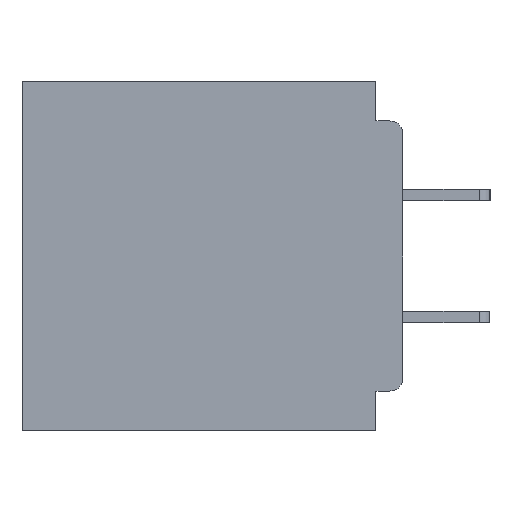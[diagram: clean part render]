
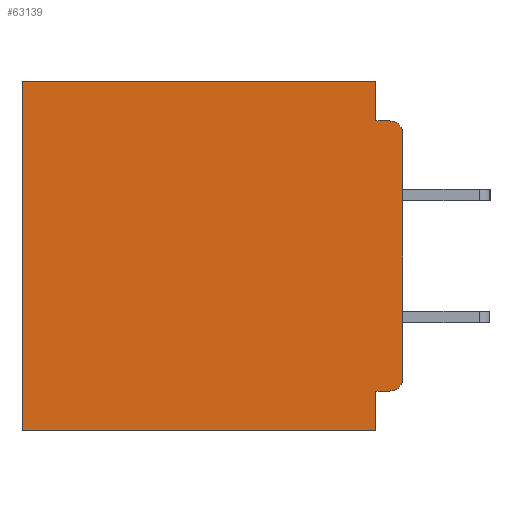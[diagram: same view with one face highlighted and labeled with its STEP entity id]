
A CAD part, left-side view. The second image highlights one B-rep face of the part: STEP entity #63139.
In plain terms, the highlighted planar face has unit normal (-1, 0, 0).
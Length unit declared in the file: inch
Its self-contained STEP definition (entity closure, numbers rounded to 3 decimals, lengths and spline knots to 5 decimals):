
#1406 = ORIENTED_EDGE ( 'NONE', *, *, #25688, .F. ) ;
#1884 = VERTEX_POINT ( 'NONE', #38710 ) ;
#3891 = VERTEX_POINT ( 'NONE', #57766 ) ;
#3892 = VERTEX_POINT ( 'NONE', #57211 ) ;
#5426 = LINE ( 'NONE', #8372, #30904 ) ;
#6672 = DIRECTION ( 'NONE',  ( 0., -1., 0. ) ) ;
#7374 = PLANE ( 'NONE',  #19209 ) ;
#7793 = DIRECTION ( 'NONE',  ( 0., 1., 0. ) ) ;
#8011 = CARTESIAN_POINT ( 'NONE',  ( 0.3, 0., 0. ) ) ;
#8372 = CARTESIAN_POINT ( 'NONE',  ( 0.3, 0., -0.4 ) ) ;
#9856 = DIRECTION ( 'NONE',  ( 0., 0., -1. ) ) ;
#10050 = EDGE_CURVE ( 'NONE', #3891, #12261, #27946, .T. ) ;
#11405 = EDGE_CURVE ( 'NONE', #1884, #25818, #19261, .T. ) ;
#12261 = VERTEX_POINT ( 'NONE', #60968 ) ;
#12792 = VECTOR ( 'NONE', #47174, 39.37008 ) ;
#12846 = EDGE_CURVE ( 'NONE', #3892, #62666, #29378, .T. ) ;
#12969 = LINE ( 'NONE', #8011, #24966 ) ;
#13209 = EDGE_CURVE ( 'NONE', #12261, #29168, #5426, .T. ) ;
#14155 = CARTESIAN_POINT ( 'NONE',  ( 0.3, 0.015, -0.06 ) ) ;
#16154 = VECTOR ( 'NONE', #48411, 39.37008 ) ;
#17164 = EDGE_CURVE ( 'NONE', #54403, #29168, #44726, .T. ) ;
#17651 = DIRECTION ( 'NONE',  ( 1., 0., 0. ) ) ;
#17861 = CARTESIAN_POINT ( 'NONE',  ( 0.3, 0., -0.355 ) ) ;
#18078 = CARTESIAN_POINT ( 'NONE',  ( 0.3, 0.437, -0.4 ) ) ;
#18871 = DIRECTION ( 'NONE',  ( 0., 1., 0. ) ) ;
#19209 = AXIS2_PLACEMENT_3D ( 'NONE', #42919, #17651, #53060 ) ;
#19261 = CIRCLE ( 'NONE', #58371, 0.015 ) ;
#19280 = ORIENTED_EDGE ( 'NONE', *, *, #13209, .F. ) ;
#19312 = DIRECTION ( 'NONE',  ( 0., 0., -1. ) ) ;
#23405 = DIRECTION ( 'NONE',  ( 0., 1., 0. ) ) ;
#24966 = VECTOR ( 'NONE', #23405, 39.37008 ) ;
#25376 = CARTESIAN_POINT ( 'NONE',  ( 0.3, 0.015, -0.34 ) ) ;
#25688 = EDGE_CURVE ( 'NONE', #3892, #3891, #58924, .T. ) ;
#25818 = VERTEX_POINT ( 'NONE', #64438 ) ;
#27182 = CARTESIAN_POINT ( 'NONE',  ( 0.3, 0.031, -0.045 ) ) ;
#27197 = LINE ( 'NONE', #27202, #39026 ) ;
#27202 = CARTESIAN_POINT ( 'NONE',  ( 0.3, 0.031, 0. ) ) ;
#27946 = LINE ( 'NONE', #52238, #12792 ) ;
#28181 = VECTOR ( 'NONE', #6672, 39.37008 ) ;
#29168 = VERTEX_POINT ( 'NONE', #59092 ) ;
#29378 = CIRCLE ( 'NONE', #41969, 0.015 ) ;
#30109 = ORIENTED_EDGE ( 'NONE', *, *, #49067, .T. ) ;
#30183 = EDGE_CURVE ( 'NONE', #36807, #25818, #46386, .T. ) ;
#30441 = DIRECTION ( 'NONE',  ( 0., 0., -1. ) ) ;
#30904 = VECTOR ( 'NONE', #18871, 39.37008 ) ;
#31365 = VECTOR ( 'NONE', #9856, 39.37008 ) ;
#36807 = VERTEX_POINT ( 'NONE', #27182 ) ;
#37076 = ORIENTED_EDGE ( 'NONE', *, *, #30183, .F. ) ;
#38710 = CARTESIAN_POINT ( 'NONE',  ( 0.3, 0., -0.06 ) ) ;
#39026 = VECTOR ( 'NONE', #47306, 39.37008 ) ;
#39165 = ORIENTED_EDGE ( 'NONE', *, *, #11405, .T. ) ;
#41969 = AXIS2_PLACEMENT_3D ( 'NONE', #25376, #60666, #30441 ) ;
#42558 = FACE_OUTER_BOUND ( 'NONE', #61421, .T. ) ;
#42919 = CARTESIAN_POINT ( 'NONE',  ( 0.3, 0., -0.4 ) ) ;
#43772 = ORIENTED_EDGE ( 'NONE', *, *, #17164, .T. ) ;
#43924 = VECTOR ( 'NONE', #7793, 39.37008 ) ;
#44726 = LINE ( 'NONE', #18078, #16154 ) ;
#44855 = CARTESIAN_POINT ( 'NONE',  ( 0.3, 0.031, 0. ) ) ;
#46386 = LINE ( 'NONE', #52137, #28181 ) ;
#47174 = DIRECTION ( 'NONE',  ( 0., 0., -1. ) ) ;
#47306 = DIRECTION ( 'NONE',  ( 0., 0., -1. ) ) ;
#48411 = DIRECTION ( 'NONE',  ( 0., 0., -1. ) ) ;
#48571 = EDGE_CURVE ( 'NONE', #1884, #62666, #58193, .T. ) ;
#49067 = EDGE_CURVE ( 'NONE', #61332, #54403, #12969, .T. ) ;
#49595 = DIRECTION ( 'NONE',  ( -1., 0., 0. ) ) ;
#50812 = EDGE_CURVE ( 'NONE', #61332, #36807, #27197, .T. ) ;
#52137 = CARTESIAN_POINT ( 'NONE',  ( 0.3, 0., -0.045 ) ) ;
#52238 = CARTESIAN_POINT ( 'NONE',  ( 0.3, 0.031, -0.4 ) ) ;
#53060 = DIRECTION ( 'NONE',  ( 0., 0., -1. ) ) ;
#53084 = ORIENTED_EDGE ( 'NONE', *, *, #48571, .F. ) ;
#54403 = VERTEX_POINT ( 'NONE', #59574 ) ;
#55157 = ORIENTED_EDGE ( 'NONE', *, *, #10050, .F. ) ;
#57211 = CARTESIAN_POINT ( 'NONE',  ( 0.3, 0.015, -0.355 ) ) ;
#57766 = CARTESIAN_POINT ( 'NONE',  ( 0.3, 0.031, -0.355 ) ) ;
#58001 = ORIENTED_EDGE ( 'NONE', *, *, #12846, .T. ) ;
#58193 = LINE ( 'NONE', #60113, #31365 ) ;
#58371 = AXIS2_PLACEMENT_3D ( 'NONE', #14155, #49595, #19312 ) ;
#58924 = LINE ( 'NONE', #17861, #43924 ) ;
#59092 = CARTESIAN_POINT ( 'NONE',  ( 0.3, 0.437, -0.4 ) ) ;
#59574 = CARTESIAN_POINT ( 'NONE',  ( 0.3, 0.437, 0. ) ) ;
#60113 = CARTESIAN_POINT ( 'NONE',  ( 0.3, 0., -0.4 ) ) ;
#60543 = CARTESIAN_POINT ( 'NONE',  ( 0.3, 0., -0.34 ) ) ;
#60666 = DIRECTION ( 'NONE',  ( -1., 0., 0. ) ) ;
#60968 = CARTESIAN_POINT ( 'NONE',  ( 0.3, 0.031, -0.4 ) ) ;
#61332 = VERTEX_POINT ( 'NONE', #44855 ) ;
#61421 = EDGE_LOOP ( 'NONE', ( #53084, #39165, #37076, #62845, #30109, #43772, #19280, #55157, #1406, #58001 ) ) ;
#62666 = VERTEX_POINT ( 'NONE', #60543 ) ;
#62845 = ORIENTED_EDGE ( 'NONE', *, *, #50812, .F. ) ;
#63139 = ADVANCED_FACE ( 'NONE', ( #42558 ), #7374, .F. ) ;
#64438 = CARTESIAN_POINT ( 'NONE',  ( 0.3, 0.015, -0.045 ) ) ;
